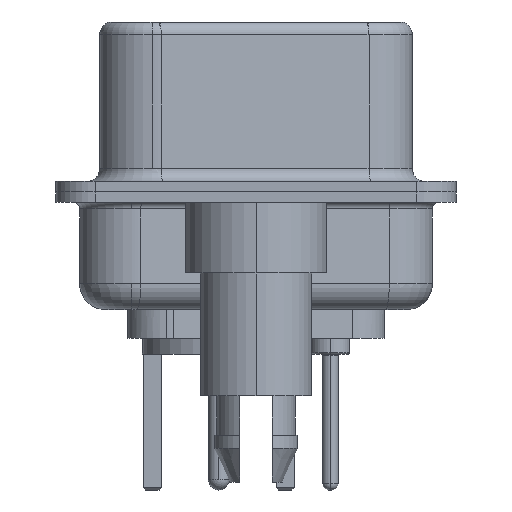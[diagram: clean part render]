
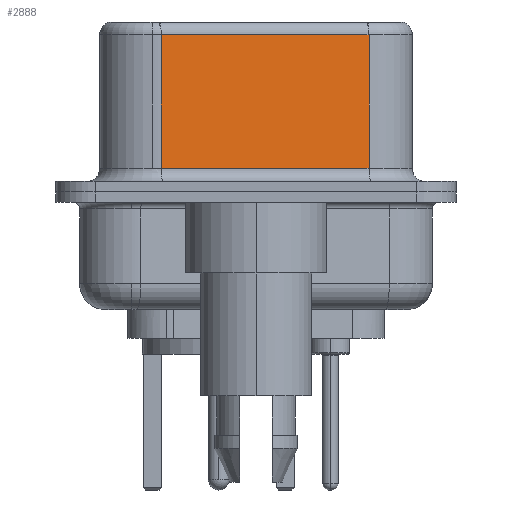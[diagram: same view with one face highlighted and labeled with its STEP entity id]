
A CAD part, left-side view. The second image highlights one B-rep face of the part: STEP entity #2888.
In plain terms, the highlighted planar face has unit normal (-0.985, -0.174, 0).
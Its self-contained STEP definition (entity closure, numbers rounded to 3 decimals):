
#2071 = CARTESIAN_POINT ( 'NONE',  ( 5.132, -4.322, 6.02 ) ) ;
#2294 = VERTEX_POINT ( 'NONE', #18676 ) ;
#2368 = ORIENTED_EDGE ( 'NONE', *, *, #15401, .T. ) ;
#2382 = DIRECTION ( 'NONE',  ( 0.174, -0.985, 0. ) ) ;
#2888 = ADVANCED_FACE ( 'NONE', ( #13532 ), #5552, .F. ) ;
#4210 = CARTESIAN_POINT ( 'NONE',  ( 3.73, 3.628, 6.52 ) ) ;
#4373 = DIRECTION ( 'NONE',  ( 0.985, 0.174, 0. ) ) ;
#5552 = PLANE ( 'NONE',  #20805 ) ;
#6004 = ORIENTED_EDGE ( 'NONE', *, *, #6850, .T. ) ;
#6202 = DIRECTION ( 'NONE',  ( 0., 0., -1. ) ) ;
#6211 = ORIENTED_EDGE ( 'NONE', *, *, #9471, .F. ) ;
#6606 = CARTESIAN_POINT ( 'NONE',  ( 5.132, -4.322, 6.52 ) ) ;
#6850 = EDGE_CURVE ( 'NONE', #20895, #16732, #12891, .T. ) ;
#8417 = VERTEX_POINT ( 'NONE', #20785 ) ;
#9149 = VECTOR ( 'NONE', #2382, 1000. ) ;
#9366 = EDGE_LOOP ( 'NONE', ( #6211, #6004, #20087, #2368 ) ) ;
#9369 = DIRECTION ( 'NONE',  ( -0.174, 0.985, 0. ) ) ;
#9471 = EDGE_CURVE ( 'NONE', #20895, #8417, #17151, .T. ) ;
#10099 = CARTESIAN_POINT ( 'NONE',  ( 5.132, -4.322, 0.9 ) ) ;
#11431 = CARTESIAN_POINT ( 'NONE',  ( 5.132, -4.322, 6.02 ) ) ;
#12027 = EDGE_CURVE ( 'NONE', #16732, #2294, #15280, .T. ) ;
#12830 = DIRECTION ( 'NONE',  ( 0., 0., -1. ) ) ;
#12891 = LINE ( 'NONE', #11431, #17267 ) ;
#12930 = CARTESIAN_POINT ( 'NONE',  ( 5.132, -4.322, 6.52 ) ) ;
#13532 = FACE_OUTER_BOUND ( 'NONE', #9366, .T. ) ;
#14254 = LINE ( 'NONE', #10099, #9149 ) ;
#15280 = LINE ( 'NONE', #4210, #23962 ) ;
#15401 = EDGE_CURVE ( 'NONE', #2294, #8417, #14254, .T. ) ;
#16196 = CARTESIAN_POINT ( 'NONE',  ( 3.73, 3.628, 6.02 ) ) ;
#16732 = VERTEX_POINT ( 'NONE', #16196 ) ;
#17151 = LINE ( 'NONE', #12930, #21474 ) ;
#17267 = VECTOR ( 'NONE', #9369, 1000. ) ;
#18676 = CARTESIAN_POINT ( 'NONE',  ( 3.73, 3.628, 0.9 ) ) ;
#20087 = ORIENTED_EDGE ( 'NONE', *, *, #12027, .T. ) ;
#20785 = CARTESIAN_POINT ( 'NONE',  ( 5.132, -4.322, 0.9 ) ) ;
#20805 = AXIS2_PLACEMENT_3D ( 'NONE', #6606, #4373, #21916 ) ;
#20895 = VERTEX_POINT ( 'NONE', #2071 ) ;
#21474 = VECTOR ( 'NONE', #12830, 1000. ) ;
#21916 = DIRECTION ( 'NONE',  ( -0.174, 0.985, 0. ) ) ;
#23962 = VECTOR ( 'NONE', #6202, 1000. ) ;
